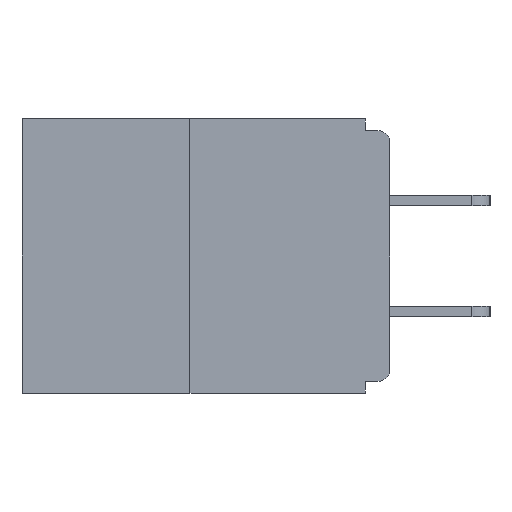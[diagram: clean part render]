
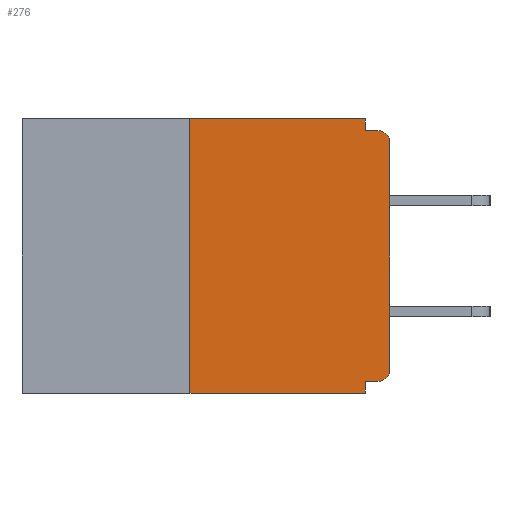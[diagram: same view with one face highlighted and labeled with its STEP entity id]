
A CAD part, left-side view. The second image highlights one B-rep face of the part: STEP entity #276.
In plain terms, the highlighted planar face has unit normal (-1, 0, 0).
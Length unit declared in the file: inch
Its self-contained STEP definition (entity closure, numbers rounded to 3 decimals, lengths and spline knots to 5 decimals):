
#194 = CARTESIAN_POINT ( 'NONE',  ( 0., 0.031, -0.015 ) ) ;
#202 = EDGE_CURVE ( 'NONE', #10372, #12825, #602, .T. ) ;
#276 = ADVANCED_FACE ( 'NONE', ( #3312 ), #12359, .F. ) ;
#330 = AXIS2_PLACEMENT_3D ( 'NONE', #1939, #8892, #1873 ) ;
#602 = LINE ( 'NONE', #2862, #7612 ) ;
#1049 = ORIENTED_EDGE ( 'NONE', *, *, #9145, .F. ) ;
#1513 = CIRCLE ( 'NONE', #12451, 0.015 ) ;
#1541 = DIRECTION ( 'NONE',  ( 0., 0., -1. ) ) ;
#1712 = ORIENTED_EDGE ( 'NONE', *, *, #4531, .T. ) ;
#1808 = DIRECTION ( 'NONE',  ( 0., 1., 0. ) ) ;
#1873 = DIRECTION ( 'NONE',  ( 0., 0., -1. ) ) ;
#1929 = EDGE_CURVE ( 'NONE', #14145, #4238, #11466, .T. ) ;
#1932 = DIRECTION ( 'NONE',  ( 0., 0., 1. ) ) ;
#1939 = CARTESIAN_POINT ( 'NONE',  ( 0., 0.46, 0. ) ) ;
#1943 = VECTOR ( 'NONE', #1808, 39.37008 ) ;
#2593 = ORIENTED_EDGE ( 'NONE', *, *, #202, .F. ) ;
#2716 = VECTOR ( 'NONE', #5820, 39.37008 ) ;
#2718 = DIRECTION ( 'NONE',  ( 0., -1., 0. ) ) ;
#2722 = EDGE_CURVE ( 'NONE', #3107, #14285, #1513, .T. ) ;
#2862 = CARTESIAN_POINT ( 'NONE',  ( 0., 0.031, -0.343 ) ) ;
#3107 = VERTEX_POINT ( 'NONE', #12278 ) ;
#3126 = CARTESIAN_POINT ( 'NONE',  ( 0., 0., -0.313 ) ) ;
#3312 = FACE_OUTER_BOUND ( 'NONE', #3868, .T. ) ;
#3330 = ORIENTED_EDGE ( 'NONE', *, *, #4806, .T. ) ;
#3464 = CARTESIAN_POINT ( 'NONE',  ( 0., 0., -0.015 ) ) ;
#3654 = DIRECTION ( 'NONE',  ( -1., 0., 0. ) ) ;
#3681 = CARTESIAN_POINT ( 'NONE',  ( 0., 0.46, -0.343 ) ) ;
#3793 = CARTESIAN_POINT ( 'NONE',  ( 0., 0.031, -0.343 ) ) ;
#3868 = EDGE_LOOP ( 'NONE', ( #10120, #6148, #1712, #2593, #12080, #5780, #6439, #3330, #5901, #1049 ) ) ;
#3929 = CARTESIAN_POINT ( 'NONE',  ( 0., 0.031, 0. ) ) ;
#4040 = DIRECTION ( 'NONE',  ( 0., 0., 1. ) ) ;
#4062 = DIRECTION ( 'NONE',  ( 0., 0., -1. ) ) ;
#4218 = LINE ( 'NONE', #8887, #12689 ) ;
#4238 = VERTEX_POINT ( 'NONE', #5927 ) ;
#4488 = VERTEX_POINT ( 'NONE', #13424 ) ;
#4531 = EDGE_CURVE ( 'NONE', #5652, #12825, #7126, .T. ) ;
#4806 = EDGE_CURVE ( 'NONE', #13691, #4238, #5869, .T. ) ;
#5135 = CARTESIAN_POINT ( 'NONE',  ( 0., 0.46, 0. ) ) ;
#5533 = DIRECTION ( 'NONE',  ( -1., 0., 0. ) ) ;
#5652 = VERTEX_POINT ( 'NONE', #13167 ) ;
#5780 = ORIENTED_EDGE ( 'NONE', *, *, #2722, .T. ) ;
#5820 = DIRECTION ( 'NONE',  ( 0., -1., 0. ) ) ;
#5869 = CIRCLE ( 'NONE', #11218, 0.015 ) ;
#5882 = CARTESIAN_POINT ( 'NONE',  ( 0., 0.015, -0.313 ) ) ;
#5901 = ORIENTED_EDGE ( 'NONE', *, *, #1929, .F. ) ;
#5927 = CARTESIAN_POINT ( 'NONE',  ( 0., 0.015, -0.015 ) ) ;
#5959 = EDGE_CURVE ( 'NONE', #4488, #11393, #14462, .T. ) ;
#6064 = EDGE_CURVE ( 'NONE', #3107, #10372, #10708, .T. ) ;
#6148 = ORIENTED_EDGE ( 'NONE', *, *, #6598, .F. ) ;
#6439 = ORIENTED_EDGE ( 'NONE', *, *, #15034, .T. ) ;
#6598 = EDGE_CURVE ( 'NONE', #5652, #4488, #14686, .T. ) ;
#7126 = LINE ( 'NONE', #3681, #10720 ) ;
#7504 = DIRECTION ( 'NONE',  ( 0., 0., -1. ) ) ;
#7612 = VECTOR ( 'NONE', #7504, 39.37008 ) ;
#8836 = DIRECTION ( 'NONE',  ( 0., 0., -1. ) ) ;
#8887 = CARTESIAN_POINT ( 'NONE',  ( 0., 0., 0. ) ) ;
#8892 = DIRECTION ( 'NONE',  ( 1., 0., 0. ) ) ;
#9145 = EDGE_CURVE ( 'NONE', #11393, #14145, #9714, .T. ) ;
#9714 = LINE ( 'NONE', #3929, #14228 ) ;
#9717 = VECTOR ( 'NONE', #4040, 39.37008 ) ;
#10015 = CARTESIAN_POINT ( 'NONE',  ( 0., 0.015, -0.03 ) ) ;
#10018 = CARTESIAN_POINT ( 'NONE',  ( 0., 0., -0.328 ) ) ;
#10120 = ORIENTED_EDGE ( 'NONE', *, *, #5959, .F. ) ;
#10347 = CARTESIAN_POINT ( 'NONE',  ( 0., 0., -0.03 ) ) ;
#10372 = VERTEX_POINT ( 'NONE', #10751 ) ;
#10708 = LINE ( 'NONE', #10018, #1943 ) ;
#10720 = VECTOR ( 'NONE', #11751, 39.37008 ) ;
#10751 = CARTESIAN_POINT ( 'NONE',  ( 0., 0.031, -0.328 ) ) ;
#10928 = VECTOR ( 'NONE', #2718, 39.37008 ) ;
#10935 = CARTESIAN_POINT ( 'NONE',  ( 0., 0.031, 0. ) ) ;
#11218 = AXIS2_PLACEMENT_3D ( 'NONE', #10015, #5533, #4062 ) ;
#11393 = VERTEX_POINT ( 'NONE', #10935 ) ;
#11466 = LINE ( 'NONE', #3464, #2716 ) ;
#11751 = DIRECTION ( 'NONE',  ( 0., -1., 0. ) ) ;
#12080 = ORIENTED_EDGE ( 'NONE', *, *, #6064, .F. ) ;
#12278 = CARTESIAN_POINT ( 'NONE',  ( 0., 0.015, -0.328 ) ) ;
#12359 = PLANE ( 'NONE',  #330 ) ;
#12451 = AXIS2_PLACEMENT_3D ( 'NONE', #5882, #3654, #1541 ) ;
#12689 = VECTOR ( 'NONE', #1932, 39.37008 ) ;
#12825 = VERTEX_POINT ( 'NONE', #3793 ) ;
#13167 = CARTESIAN_POINT ( 'NONE',  ( 0., 0.25, -0.343 ) ) ;
#13424 = CARTESIAN_POINT ( 'NONE',  ( 0., 0.25, 0. ) ) ;
#13691 = VERTEX_POINT ( 'NONE', #10347 ) ;
#14145 = VERTEX_POINT ( 'NONE', #194 ) ;
#14228 = VECTOR ( 'NONE', #8836, 39.37008 ) ;
#14285 = VERTEX_POINT ( 'NONE', #3126 ) ;
#14462 = LINE ( 'NONE', #5135, #10928 ) ;
#14686 = LINE ( 'NONE', #14762, #9717 ) ;
#14762 = CARTESIAN_POINT ( 'NONE',  ( 0., 0.25, 0. ) ) ;
#15034 = EDGE_CURVE ( 'NONE', #14285, #13691, #4218, .T. ) ;
